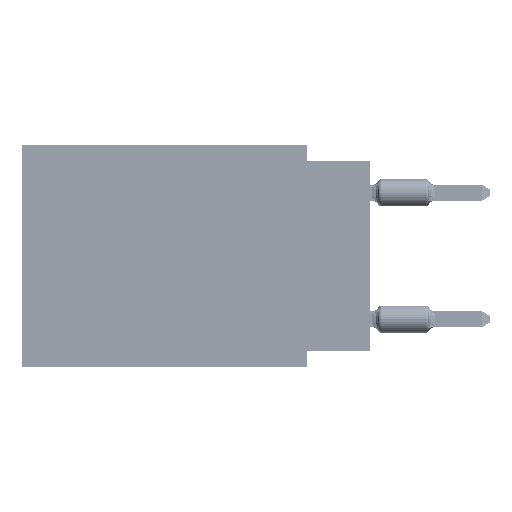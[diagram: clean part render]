
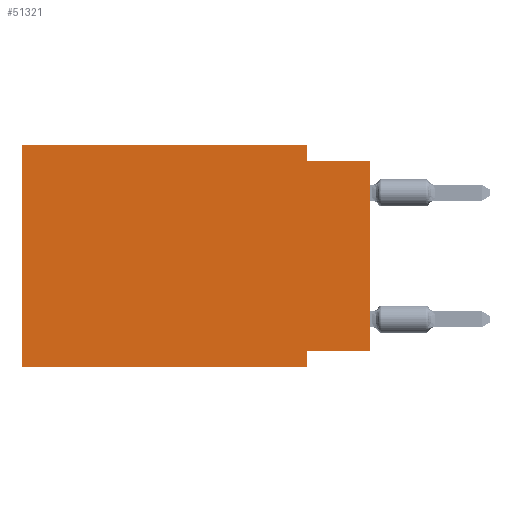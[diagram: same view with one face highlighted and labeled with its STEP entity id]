
A CAD part, left-side view. The second image highlights one B-rep face of the part: STEP entity #51321.
In plain terms, the highlighted planar face has unit normal (-1, 0, 0).
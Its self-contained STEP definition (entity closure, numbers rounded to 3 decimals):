
#792 = VECTOR ( 'NONE', #64874, 1000. ) ;
#1945 = VERTEX_POINT ( 'NONE', #81145 ) ;
#3049 = DIRECTION ( 'NONE',  ( 0., 0., -1. ) ) ;
#3117 = CARTESIAN_POINT ( 'NONE',  ( 0., 2.54, 0. ) ) ;
#3481 = AXIS2_PLACEMENT_3D ( 'NONE', #70855, #31508, #25496 ) ;
#5384 = FACE_OUTER_BOUND ( 'NONE', #62409, .T. ) ;
#5563 = EDGE_CURVE ( 'NONE', #31978, #60734, #44798, .T. ) ;
#8452 = DIRECTION ( 'NONE',  ( 0., -1., 0. ) ) ;
#9068 = LINE ( 'NONE', #59589, #19469 ) ;
#9745 = VECTOR ( 'NONE', #8452, 1000. ) ;
#11559 = LINE ( 'NONE', #37665, #45272 ) ;
#12276 = LINE ( 'NONE', #69625, #78750 ) ;
#12467 = CARTESIAN_POINT ( 'NONE',  ( 0., 2.54, 0. ) ) ;
#16336 = LINE ( 'NONE', #54849, #35073 ) ;
#16602 = LINE ( 'NONE', #82476, #792 ) ;
#18196 = EDGE_CURVE ( 'NONE', #1945, #78821, #16602, .T. ) ;
#18248 = EDGE_CURVE ( 'NONE', #78821, #34418, #12276, .T. ) ;
#18780 = CARTESIAN_POINT ( 'NONE',  ( 0., 2.54, -0.635 ) ) ;
#19469 = VECTOR ( 'NONE', #35179, 1000. ) ;
#23633 = CARTESIAN_POINT ( 'NONE',  ( 0., 13.97, 0. ) ) ;
#25496 = DIRECTION ( 'NONE',  ( 0., 0., -1. ) ) ;
#26452 = CARTESIAN_POINT ( 'NONE',  ( 0., 0., -8.255 ) ) ;
#29392 = ORIENTED_EDGE ( 'NONE', *, *, #32111, .T. ) ;
#30058 = EDGE_CURVE ( 'NONE', #34418, #58044, #61751, .T. ) ;
#31255 = DIRECTION ( 'NONE',  ( 0., 1., 0. ) ) ;
#31508 = DIRECTION ( 'NONE',  ( 1., 0., 0. ) ) ;
#31957 = CARTESIAN_POINT ( 'NONE',  ( 0., 0., 0. ) ) ;
#31978 = VERTEX_POINT ( 'NONE', #26452 ) ;
#32111 = EDGE_CURVE ( 'NONE', #1945, #66722, #40986, .T. ) ;
#32453 = ORIENTED_EDGE ( 'NONE', *, *, #18196, .F. ) ;
#34418 = VERTEX_POINT ( 'NONE', #12467 ) ;
#35073 = VECTOR ( 'NONE', #3049, 1000. ) ;
#35179 = DIRECTION ( 'NONE',  ( 0., -1., 0. ) ) ;
#37391 = VECTOR ( 'NONE', #57637, 1000. ) ;
#37665 = CARTESIAN_POINT ( 'NONE',  ( 0., 0., -8.255 ) ) ;
#40986 = LINE ( 'NONE', #67075, #9745 ) ;
#44798 = LINE ( 'NONE', #31957, #37391 ) ;
#45272 = VECTOR ( 'NONE', #31255, 1000. ) ;
#46290 = VERTEX_POINT ( 'NONE', #84525 ) ;
#49040 = EDGE_CURVE ( 'NONE', #58044, #60734, #9068, .T. ) ;
#50766 = PLANE ( 'NONE',  #3481 ) ;
#51321 = ADVANCED_FACE ( 'NONE', ( #5384 ), #50766, .F. ) ;
#54034 = ORIENTED_EDGE ( 'NONE', *, *, #72241, .F. ) ;
#54849 = CARTESIAN_POINT ( 'NONE',  ( 0., 2.54, -8.89 ) ) ;
#55661 = EDGE_CURVE ( 'NONE', #31978, #46290, #11559, .T. ) ;
#56186 = DIRECTION ( 'NONE',  ( 0., 0., -1. ) ) ;
#56380 = DIRECTION ( 'NONE',  ( 0., -1., 0. ) ) ;
#56520 = ORIENTED_EDGE ( 'NONE', *, *, #18248, .F. ) ;
#57637 = DIRECTION ( 'NONE',  ( 0., 0., 1. ) ) ;
#57997 = CARTESIAN_POINT ( 'NONE',  ( 0., 2.54, -8.89 ) ) ;
#58044 = VERTEX_POINT ( 'NONE', #18780 ) ;
#59336 = ORIENTED_EDGE ( 'NONE', *, *, #30058, .F. ) ;
#59589 = CARTESIAN_POINT ( 'NONE',  ( 0., 0., -0.635 ) ) ;
#60734 = VERTEX_POINT ( 'NONE', #64860 ) ;
#61751 = LINE ( 'NONE', #3117, #79397 ) ;
#62286 = ORIENTED_EDGE ( 'NONE', *, *, #55661, .F. ) ;
#62409 = EDGE_LOOP ( 'NONE', ( #74253, #82866, #59336, #56520, #32453, #29392, #54034, #62286 ) ) ;
#64860 = CARTESIAN_POINT ( 'NONE',  ( 0., 0., -0.635 ) ) ;
#64874 = DIRECTION ( 'NONE',  ( 0., 0., 1. ) ) ;
#66722 = VERTEX_POINT ( 'NONE', #57997 ) ;
#67075 = CARTESIAN_POINT ( 'NONE',  ( 0., 13.97, -8.89 ) ) ;
#69625 = CARTESIAN_POINT ( 'NONE',  ( 0., 13.97, 0. ) ) ;
#70855 = CARTESIAN_POINT ( 'NONE',  ( 0., 13.97, 0. ) ) ;
#72241 = EDGE_CURVE ( 'NONE', #46290, #66722, #16336, .T. ) ;
#74253 = ORIENTED_EDGE ( 'NONE', *, *, #5563, .T. ) ;
#78750 = VECTOR ( 'NONE', #56380, 1000. ) ;
#78821 = VERTEX_POINT ( 'NONE', #23633 ) ;
#79397 = VECTOR ( 'NONE', #56186, 1000. ) ;
#81145 = CARTESIAN_POINT ( 'NONE',  ( 0., 13.97, -8.89 ) ) ;
#82476 = CARTESIAN_POINT ( 'NONE',  ( 0., 13.97, 0. ) ) ;
#82866 = ORIENTED_EDGE ( 'NONE', *, *, #49040, .F. ) ;
#84525 = CARTESIAN_POINT ( 'NONE',  ( 0., 2.54, -8.255 ) ) ;
